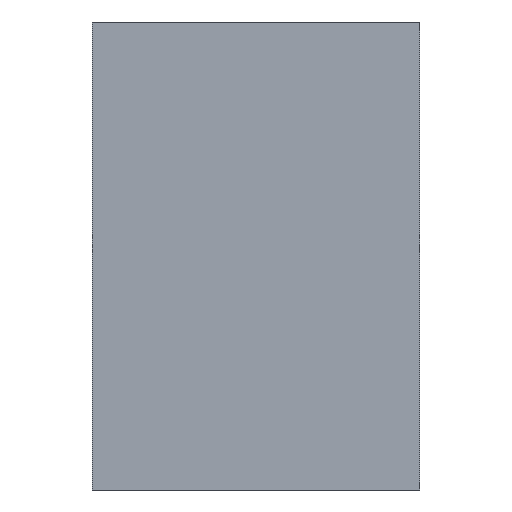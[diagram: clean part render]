
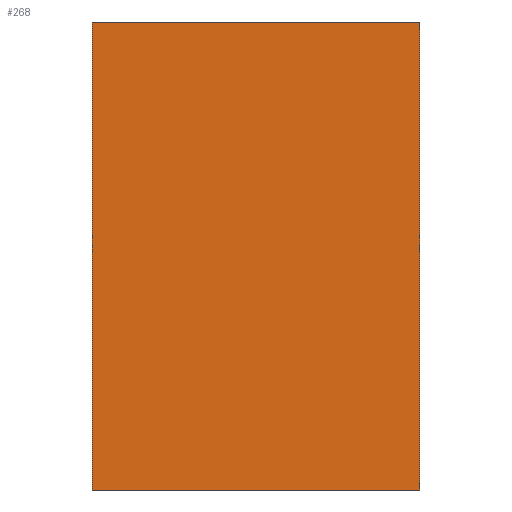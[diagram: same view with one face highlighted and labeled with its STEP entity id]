
A CAD part, left-side view. The second image highlights one B-rep face of the part: STEP entity #268.
In plain terms, the highlighted planar face has unit normal (-1, 0, 0).
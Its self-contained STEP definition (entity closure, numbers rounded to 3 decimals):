
#23 = VERTEX_POINT ( 'NONE', #254 ) ;
#36 = FACE_OUTER_BOUND ( 'NONE', #287, .T. ) ;
#68 = AXIS2_PLACEMENT_3D ( 'NONE', #523, #311, #468 ) ;
#81 = DIRECTION ( 'NONE',  ( 0., 0., -1. ) ) ;
#84 = VECTOR ( 'NONE', #219, 1000. ) ;
#87 = ORIENTED_EDGE ( 'NONE', *, *, #487, .T. ) ;
#89 = DIRECTION ( 'NONE',  ( 0., -1., 0. ) ) ;
#134 = EDGE_CURVE ( 'NONE', #282, #151, #352, .T. ) ;
#151 = VERTEX_POINT ( 'NONE', #366 ) ;
#163 = VECTOR ( 'NONE', #573, 1000. ) ;
#183 = CARTESIAN_POINT ( 'NONE',  ( 0., 0., 0. ) ) ;
#203 = VERTEX_POINT ( 'NONE', #629 ) ;
#212 = PLANE ( 'NONE',  #68 ) ;
#213 = CARTESIAN_POINT ( 'NONE',  ( 0., -5., 10. ) ) ;
#219 = DIRECTION ( 'NONE',  ( 0., 0., 1. ) ) ;
#249 = LINE ( 'NONE', #529, #84 ) ;
#254 = CARTESIAN_POINT ( 'NONE',  ( 0., 2., 0. ) ) ;
#268 = ADVANCED_FACE ( 'NONE', ( #36 ), #212, .F. ) ;
#282 = VERTEX_POINT ( 'NONE', #518 ) ;
#287 = EDGE_LOOP ( 'NONE', ( #87, #613, #433, #570 ) ) ;
#311 = DIRECTION ( 'NONE',  ( 1., 0., 0. ) ) ;
#340 = EDGE_CURVE ( 'NONE', #23, #282, #249, .T. ) ;
#351 = VECTOR ( 'NONE', #81, 1000. ) ;
#352 = LINE ( 'NONE', #410, #163 ) ;
#353 = EDGE_CURVE ( 'NONE', #151, #203, #560, .T. ) ;
#356 = LINE ( 'NONE', #183, #540 ) ;
#366 = CARTESIAN_POINT ( 'NONE',  ( 0., -5., 10. ) ) ;
#410 = CARTESIAN_POINT ( 'NONE',  ( 0., 0., 10. ) ) ;
#433 = ORIENTED_EDGE ( 'NONE', *, *, #134, .F. ) ;
#468 = DIRECTION ( 'NONE',  ( 0., 0., -1. ) ) ;
#487 = EDGE_CURVE ( 'NONE', #23, #203, #356, .T. ) ;
#518 = CARTESIAN_POINT ( 'NONE',  ( 0., 2., 10. ) ) ;
#523 = CARTESIAN_POINT ( 'NONE',  ( 0., 0., 10. ) ) ;
#529 = CARTESIAN_POINT ( 'NONE',  ( 0., 2., 0. ) ) ;
#540 = VECTOR ( 'NONE', #89, 1000. ) ;
#560 = LINE ( 'NONE', #213, #351 ) ;
#570 = ORIENTED_EDGE ( 'NONE', *, *, #340, .F. ) ;
#573 = DIRECTION ( 'NONE',  ( 0., -1., 0. ) ) ;
#613 = ORIENTED_EDGE ( 'NONE', *, *, #353, .F. ) ;
#629 = CARTESIAN_POINT ( 'NONE',  ( 0., -5., 0. ) ) ;
